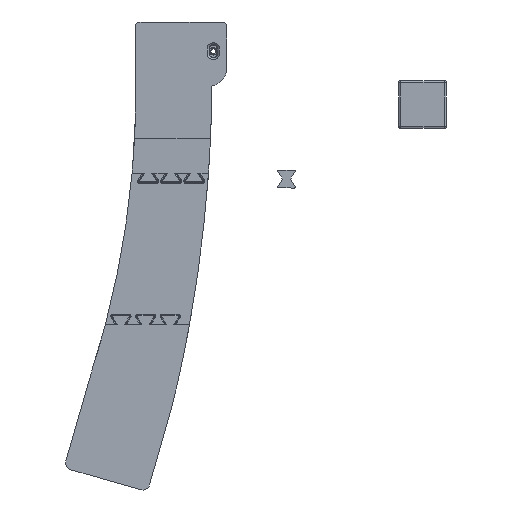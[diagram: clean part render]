
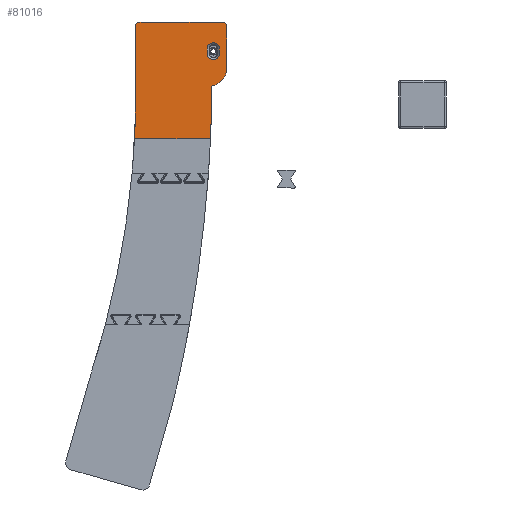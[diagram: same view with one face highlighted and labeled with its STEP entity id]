
A CAD part, front view. The second image highlights one B-rep face of the part: STEP entity #81016.
In plain terms, the highlighted planar face has unit normal (0, -1, 0).
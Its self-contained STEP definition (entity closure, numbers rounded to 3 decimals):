
#6768=FACE_BOUND('',#30846,.T.);
#7696=PLANE('',#83800);
#8501=LINE('',#98447,#14556);
#9068=LINE('',#101335,#15123);
#12443=LINE('',#148022,#18498);
#12444=LINE('',#148025,#18499);
#12445=LINE('',#148029,#18500);
#12446=LINE('',#148032,#18501);
#12447=LINE('',#148036,#18502);
#14556=VECTOR('',#85867,10.);
#15123=VECTOR('',#86786,10.);
#18498=VECTOR('',#92307,10.);
#18499=VECTOR('',#92310,10.);
#18500=VECTOR('',#92315,10.);
#18501=VECTOR('',#92316,10.);
#18502=VECTOR('',#92319,10.);
#26069=FACE_OUTER_BOUND('',#30845,.T.);
#30845=EDGE_LOOP('',(#71534,#71535,#71536,#71537,#71538,#71539,#71540,#71541,
#71542,#71543));
#30846=EDGE_LOOP('',(#71544,#71545,#71546,#71547));
#32311=CIRCLE('',#83758,949.);
#32326=CIRCLE('',#83785,1465.281);
#32327=CIRCLE('',#83801,5.);
#32328=CIRCLE('',#83802,20.);
#32329=CIRCLE('',#83803,5.);
#32330=CIRCLE('',#83804,6.439);
#32331=CIRCLE('',#83805,6.439);
#32939=VERTEX_POINT('',#98445);
#32940=VERTEX_POINT('',#98446);
#33461=VERTEX_POINT('',#101331);
#33463=VERTEX_POINT('',#101334);
#38715=VERTEX_POINT('',#147630);
#38744=VERTEX_POINT('',#147990);
#38745=VERTEX_POINT('',#148020);
#38746=VERTEX_POINT('',#148021);
#38747=VERTEX_POINT('',#148023);
#38748=VERTEX_POINT('',#148027);
#38749=VERTEX_POINT('',#148030);
#38750=VERTEX_POINT('',#148031);
#38751=VERTEX_POINT('',#148033);
#38752=VERTEX_POINT('',#148035);
#41244=EDGE_CURVE('',#32939,#32940,#8501,.T.);
#42023=EDGE_CURVE('',#33461,#33463,#9068,.T.);
#49934=EDGE_CURVE('',#38715,#32939,#32311,.T.);
#49980=EDGE_CURVE('',#32940,#38744,#32326,.T.);
#49993=EDGE_CURVE('',#38745,#38746,#12443,.T.);
#49994=EDGE_CURVE('',#38747,#38745,#32327,.T.);
#49995=EDGE_CURVE('',#38747,#38715,#12444,.T.);
#49996=EDGE_CURVE('',#33463,#38744,#32328,.T.);
#49997=EDGE_CURVE('',#38748,#33461,#32329,.T.);
#49998=EDGE_CURVE('',#38746,#38748,#12445,.T.);
#49999=EDGE_CURVE('',#38749,#38750,#12446,.T.);
#50000=EDGE_CURVE('',#38750,#38751,#32330,.T.);
#50001=EDGE_CURVE('',#38751,#38752,#12447,.T.);
#50002=EDGE_CURVE('',#38752,#38749,#32331,.T.);
#71534=ORIENTED_EDGE('',*,*,#49993,.F.);
#71535=ORIENTED_EDGE('',*,*,#49994,.F.);
#71536=ORIENTED_EDGE('',*,*,#49995,.T.);
#71537=ORIENTED_EDGE('',*,*,#49934,.T.);
#71538=ORIENTED_EDGE('',*,*,#41244,.T.);
#71539=ORIENTED_EDGE('',*,*,#49980,.T.);
#71540=ORIENTED_EDGE('',*,*,#49996,.F.);
#71541=ORIENTED_EDGE('',*,*,#42023,.F.);
#71542=ORIENTED_EDGE('',*,*,#49997,.F.);
#71543=ORIENTED_EDGE('',*,*,#49998,.F.);
#71544=ORIENTED_EDGE('',*,*,#49999,.T.);
#71545=ORIENTED_EDGE('',*,*,#50000,.T.);
#71546=ORIENTED_EDGE('',*,*,#50001,.T.);
#71547=ORIENTED_EDGE('',*,*,#50002,.T.);
#81016=ADVANCED_FACE('',(#26069,#6768),#7696,.T.);
#83758=AXIS2_PLACEMENT_3D('',#147631,#92197,#92198);
#83785=AXIS2_PLACEMENT_3D('',#147992,#92263,#92264);
#83800=AXIS2_PLACEMENT_3D('',#148019,#92305,#92306);
#83801=AXIS2_PLACEMENT_3D('',#148024,#92308,#92309);
#83802=AXIS2_PLACEMENT_3D('',#148026,#92311,#92312);
#83803=AXIS2_PLACEMENT_3D('',#148028,#92313,#92314);
#83804=AXIS2_PLACEMENT_3D('',#148034,#92317,#92318);
#83805=AXIS2_PLACEMENT_3D('',#148037,#92320,#92321);
#85867=DIRECTION('',(1.,0.,0.));
#86786=DIRECTION('',(0.,0.,-1.));
#92197=DIRECTION('center_axis',(0.,1.,0.));
#92198=DIRECTION('ref_axis',(1.,0.,-0.031));
#92263=DIRECTION('center_axis',(0.,-1.,0.));
#92264=DIRECTION('ref_axis',(1.,0.,-0.008));
#92305=DIRECTION('center_axis',(0.,-1.,0.));
#92306=DIRECTION('ref_axis',(1.,0.,0.));
#92307=DIRECTION('',(1.,0.,0.));
#92308=DIRECTION('center_axis',(0.,1.,0.));
#92309=DIRECTION('ref_axis',(-0.707,0.,0.707));
#92310=DIRECTION('',(0.,0.,-1.));
#92311=DIRECTION('center_axis',(0.,1.,0.));
#92312=DIRECTION('ref_axis',(0.208,0.,-0.978));
#92313=DIRECTION('center_axis',(0.,1.,0.));
#92314=DIRECTION('ref_axis',(0.707,0.,0.707));
#92315=DIRECTION('',(1.,0.,0.));
#92316=DIRECTION('',(0.,0.,1.));
#92317=DIRECTION('center_axis',(0.,1.,0.));
#92318=DIRECTION('ref_axis',(1.,0.,0.));
#92319=DIRECTION('',(0.,0.,-1.));
#92320=DIRECTION('center_axis',(0.,1.,0.));
#92321=DIRECTION('ref_axis',(-1.,0.,0.));
#98445=CARTESIAN_POINT('',(-101.234,6.118,-44.965));
#98446=CARTESIAN_POINT('',(-21.454,6.118,-44.965));
#98447=CARTESIAN_POINT('',(-106.432,6.118,-44.965));
#101331=CARTESIAN_POINT('',(-4.16,6.118,72.408));
#101334=CARTESIAN_POINT('',(-4.16,6.118,29.563));
#101335=CARTESIAN_POINT('',(-4.16,6.118,-37.278));
#147630=CARTESIAN_POINT('',(-100.44,6.118,-25.509));
#147631=CARTESIAN_POINT('Origin',(-1048.998,6.118,3.472));
#147990=CARTESIAN_POINT('',(-20.,6.118,10.));
#147992=CARTESIAN_POINT('Origin',(-1485.238,6.118,21.265));
#148019=CARTESIAN_POINT('Origin',(-73.595,6.118,-92.256));
#148020=CARTESIAN_POINT('',(-95.44,6.118,77.408));
#148021=CARTESIAN_POINT('',(-91.44,6.118,77.408));
#148022=CARTESIAN_POINT('',(-91.44,6.118,77.408));
#148023=CARTESIAN_POINT('',(-100.44,6.118,72.408));
#148024=CARTESIAN_POINT('Origin',(-95.44,6.118,72.408));
#148025=CARTESIAN_POINT('',(-100.44,6.118,14.491));
#148026=CARTESIAN_POINT('Origin',(-24.16,6.118,29.563));
#148027=CARTESIAN_POINT('',(-9.16,6.118,77.408));
#148028=CARTESIAN_POINT('Origin',(-9.16,6.118,72.408));
#148029=CARTESIAN_POINT('',(-9.16,6.118,77.408));
#148030=CARTESIAN_POINT('',(-24.93,6.118,44.172));
#148031=CARTESIAN_POINT('',(-24.93,6.118,49.176));
#148032=CARTESIAN_POINT('',(-24.93,6.118,65.879));
#148033=CARTESIAN_POINT('',(-12.053,6.118,49.176));
#148034=CARTESIAN_POINT('Origin',(-18.491,6.118,49.176));
#148035=CARTESIAN_POINT('',(-12.053,6.118,44.172));
#148036=CARTESIAN_POINT('',(-12.053,6.118,68.38));
#148037=CARTESIAN_POINT('Origin',(-18.491,6.118,44.172));
